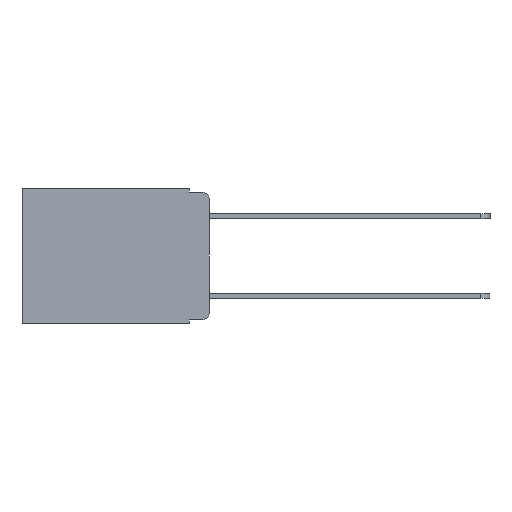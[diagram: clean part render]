
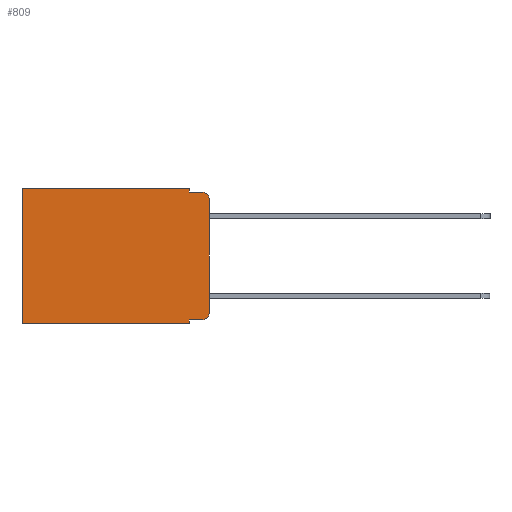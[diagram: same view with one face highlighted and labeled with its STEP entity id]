
A CAD part, left-side view. The second image highlights one B-rep face of the part: STEP entity #809.
In plain terms, the highlighted planar face has unit normal (-1, 0, 0).
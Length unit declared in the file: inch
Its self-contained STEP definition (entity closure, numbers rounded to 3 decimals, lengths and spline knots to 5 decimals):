
#23 = LINE ( 'NONE', #6992, #2234 ) ;
#50 = CARTESIAN_POINT ( 'NONE',  ( 0.298, 0.02, -0.313 ) ) ;
#416 = VERTEX_POINT ( 'NONE', #4084 ) ;
#809 = ADVANCED_FACE ( 'NONE', ( #9263 ), #4129, .F. ) ;
#997 = DIRECTION ( 'NONE',  ( 0., 0., -1. ) ) ;
#1049 = VERTEX_POINT ( 'NONE', #8550 ) ;
#1235 = LINE ( 'NONE', #7877, #7775 ) ;
#1644 = VECTOR ( 'NONE', #6478, 39.37008 ) ;
#1779 = VERTEX_POINT ( 'NONE', #10464 ) ;
#1952 = DIRECTION ( 'NONE',  ( 0., 0., -1. ) ) ;
#2003 = ORIENTED_EDGE ( 'NONE', *, *, #6286, .F. ) ;
#2234 = VECTOR ( 'NONE', #8497, 39.37008 ) ;
#2238 = CARTESIAN_POINT ( 'NONE',  ( 0.298, 0.051, -0.333 ) ) ;
#2307 = VERTEX_POINT ( 'NONE', #5475 ) ;
#2384 = CARTESIAN_POINT ( 'NONE',  ( 0.298, 0.051, -0.333 ) ) ;
#2445 = CARTESIAN_POINT ( 'NONE',  ( 0.298, 0.473, -0.343 ) ) ;
#2659 = EDGE_CURVE ( 'NONE', #7463, #1049, #5390, .T. ) ;
#2911 = DIRECTION ( 'NONE',  ( 0., 1., 0. ) ) ;
#3101 = VECTOR ( 'NONE', #8057, 39.37008 ) ;
#3331 = VECTOR ( 'NONE', #9365, 39.37008 ) ;
#3581 = AXIS2_PLACEMENT_3D ( 'NONE', #7621, #5328, #9185 ) ;
#3618 = AXIS2_PLACEMENT_3D ( 'NONE', #5115, #10481, #5931 ) ;
#3764 = ORIENTED_EDGE ( 'NONE', *, *, #5468, .T. ) ;
#3937 = ORIENTED_EDGE ( 'NONE', *, *, #4423, .F. ) ;
#3958 = ORIENTED_EDGE ( 'NONE', *, *, #5595, .F. ) ;
#4084 = CARTESIAN_POINT ( 'NONE',  ( 0.298, 0.02, -0.333 ) ) ;
#4097 = LINE ( 'NONE', #5681, #1644 ) ;
#4129 = PLANE ( 'NONE',  #3581 ) ;
#4199 = ORIENTED_EDGE ( 'NONE', *, *, #6678, .T. ) ;
#4423 = EDGE_CURVE ( 'NONE', #9748, #10065, #4562, .T. ) ;
#4562 = LINE ( 'NONE', #5709, #10495 ) ;
#4735 = VERTEX_POINT ( 'NONE', #7083 ) ;
#4782 = VERTEX_POINT ( 'NONE', #7144 ) ;
#4912 = ORIENTED_EDGE ( 'NONE', *, *, #7374, .F. ) ;
#5115 = CARTESIAN_POINT ( 'NONE',  ( 0.298, 0.02, -0.03 ) ) ;
#5328 = DIRECTION ( 'NONE',  ( 1., 0., 0. ) ) ;
#5387 = CARTESIAN_POINT ( 'NONE',  ( 0.298, 0., -0.313 ) ) ;
#5390 = LINE ( 'NONE', #6051, #3331 ) ;
#5468 = EDGE_CURVE ( 'NONE', #4735, #1779, #8937, .T. ) ;
#5475 = CARTESIAN_POINT ( 'NONE',  ( 0.298, 0.02, -0.01 ) ) ;
#5595 = EDGE_CURVE ( 'NONE', #1049, #10633, #1235, .T. ) ;
#5681 = CARTESIAN_POINT ( 'NONE',  ( 0.298, 0.051, 0. ) ) ;
#5709 = CARTESIAN_POINT ( 'NONE',  ( 0.298, 0., 0. ) ) ;
#5931 = DIRECTION ( 'NONE',  ( 0., 0., -1. ) ) ;
#6051 = CARTESIAN_POINT ( 'NONE',  ( 0.298, 0.051, 0. ) ) ;
#6217 = DIRECTION ( 'NONE',  ( 0., 0., -1. ) ) ;
#6286 = EDGE_CURVE ( 'NONE', #4782, #2307, #23, .T. ) ;
#6311 = DIRECTION ( 'NONE',  ( -1., 0., 0. ) ) ;
#6341 = ORIENTED_EDGE ( 'NONE', *, *, #6806, .T. ) ;
#6478 = DIRECTION ( 'NONE',  ( 0., 0., -1. ) ) ;
#6678 = EDGE_CURVE ( 'NONE', #7463, #416, #9490, .T. ) ;
#6806 = EDGE_CURVE ( 'NONE', #9748, #2307, #8563, .T. ) ;
#6941 = VECTOR ( 'NONE', #8510, 39.37008 ) ;
#6992 = CARTESIAN_POINT ( 'NONE',  ( 0.298, 0.051, -0.01 ) ) ;
#7083 = CARTESIAN_POINT ( 'NONE',  ( 0.298, 0.051, 0. ) ) ;
#7144 = CARTESIAN_POINT ( 'NONE',  ( 0.298, 0.051, -0.01 ) ) ;
#7183 = EDGE_CURVE ( 'NONE', #416, #10065, #9722, .T. ) ;
#7374 = EDGE_CURVE ( 'NONE', #4735, #4782, #4097, .T. ) ;
#7463 = VERTEX_POINT ( 'NONE', #2384 ) ;
#7621 = CARTESIAN_POINT ( 'NONE',  ( 0.298, 0., 0. ) ) ;
#7632 = EDGE_LOOP ( 'NONE', ( #3937, #6341, #2003, #4912, #3764, #9306, #3958, #7808, #4199, #7903 ) ) ;
#7773 = CARTESIAN_POINT ( 'NONE',  ( 0.298, 0., 0. ) ) ;
#7775 = VECTOR ( 'NONE', #2911, 39.37008 ) ;
#7808 = ORIENTED_EDGE ( 'NONE', *, *, #2659, .F. ) ;
#7855 = CARTESIAN_POINT ( 'NONE',  ( 0.298, 0.473, 0. ) ) ;
#7877 = CARTESIAN_POINT ( 'NONE',  ( 0.298, 0., -0.343 ) ) ;
#7903 = ORIENTED_EDGE ( 'NONE', *, *, #7183, .T. ) ;
#7963 = VECTOR ( 'NONE', #1952, 39.37008 ) ;
#7977 = AXIS2_PLACEMENT_3D ( 'NONE', #50, #6311, #997 ) ;
#8057 = DIRECTION ( 'NONE',  ( 0., -1., 0. ) ) ;
#8187 = LINE ( 'NONE', #7855, #7963 ) ;
#8497 = DIRECTION ( 'NONE',  ( 0., -1., 0. ) ) ;
#8510 = DIRECTION ( 'NONE',  ( 0., 1., 0. ) ) ;
#8550 = CARTESIAN_POINT ( 'NONE',  ( 0.298, 0.051, -0.343 ) ) ;
#8563 = CIRCLE ( 'NONE', #3618, 0.02 ) ;
#8910 = CARTESIAN_POINT ( 'NONE',  ( 0.298, 0., -0.03 ) ) ;
#8937 = LINE ( 'NONE', #7773, #6941 ) ;
#9185 = DIRECTION ( 'NONE',  ( 0., 0., -1. ) ) ;
#9263 = FACE_OUTER_BOUND ( 'NONE', #7632, .T. ) ;
#9306 = ORIENTED_EDGE ( 'NONE', *, *, #9370, .T. ) ;
#9365 = DIRECTION ( 'NONE',  ( 0., 0., -1. ) ) ;
#9370 = EDGE_CURVE ( 'NONE', #1779, #10633, #8187, .T. ) ;
#9490 = LINE ( 'NONE', #2238, #3101 ) ;
#9722 = CIRCLE ( 'NONE', #7977, 0.02 ) ;
#9748 = VERTEX_POINT ( 'NONE', #8910 ) ;
#10065 = VERTEX_POINT ( 'NONE', #5387 ) ;
#10464 = CARTESIAN_POINT ( 'NONE',  ( 0.298, 0.473, 0. ) ) ;
#10481 = DIRECTION ( 'NONE',  ( -1., 0., 0. ) ) ;
#10495 = VECTOR ( 'NONE', #6217, 39.37008 ) ;
#10633 = VERTEX_POINT ( 'NONE', #2445 ) ;
